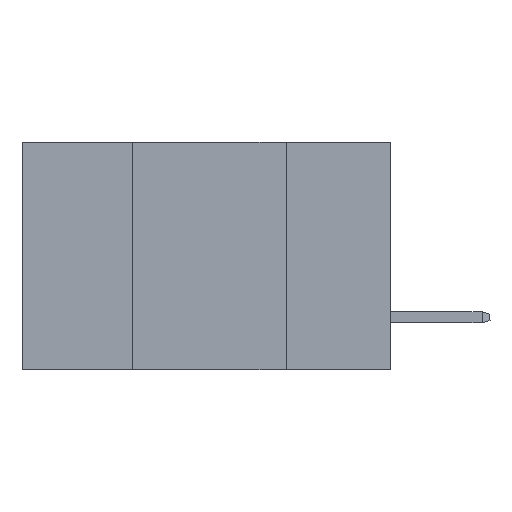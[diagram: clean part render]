
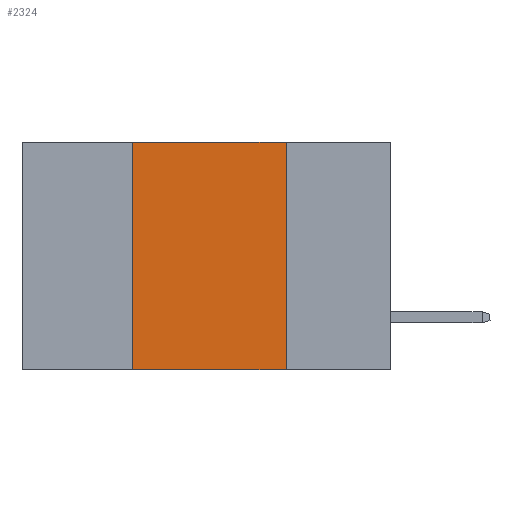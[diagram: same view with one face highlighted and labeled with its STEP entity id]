
A CAD part, left-side view. The second image highlights one B-rep face of the part: STEP entity #2324.
In plain terms, the highlighted planar face has unit normal (-1, 0, 0).
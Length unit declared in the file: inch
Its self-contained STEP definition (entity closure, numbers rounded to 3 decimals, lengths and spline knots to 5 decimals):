
#345 = VERTEX_POINT ( 'NONE', #1541 ) ;
#495 = VECTOR ( 'NONE', #648, 39.37008 ) ;
#512 = EDGE_LOOP ( 'NONE', ( #8416, #5565, #4851, #6882 ) ) ;
#648 = DIRECTION ( 'NONE',  ( 0., -1., 0. ) ) ;
#925 = CARTESIAN_POINT ( 'NONE',  ( 0., 0.17, 0. ) ) ;
#994 = CARTESIAN_POINT ( 'NONE',  ( 0., 0.42, 0. ) ) ;
#1031 = VECTOR ( 'NONE', #8140, 39.37008 ) ;
#1502 = LINE ( 'NONE', #4062, #2975 ) ;
#1541 = CARTESIAN_POINT ( 'NONE',  ( 0., 0.17, 0. ) ) ;
#1684 = VECTOR ( 'NONE', #4405, 39.37008 ) ;
#2297 = VERTEX_POINT ( 'NONE', #6514 ) ;
#2324 = ADVANCED_FACE ( 'NONE', ( #8362 ), #5560, .F. ) ;
#2580 = EDGE_CURVE ( 'NONE', #8582, #345, #1502, .T. ) ;
#2642 = CARTESIAN_POINT ( 'NONE',  ( 0., 0.6, -0.37 ) ) ;
#2975 = VECTOR ( 'NONE', #6668, 39.37008 ) ;
#3455 = EDGE_CURVE ( 'NONE', #345, #2297, #6512, .T. ) ;
#3498 = CARTESIAN_POINT ( 'NONE',  ( 0., 0.42, 0. ) ) ;
#4062 = CARTESIAN_POINT ( 'NONE',  ( 0., 0.6, 0. ) ) ;
#4255 = EDGE_CURVE ( 'NONE', #4478, #8582, #8702, .T. ) ;
#4405 = DIRECTION ( 'NONE',  ( 0., 0., 1. ) ) ;
#4478 = VERTEX_POINT ( 'NONE', #7391 ) ;
#4806 = AXIS2_PLACEMENT_3D ( 'NONE', #6916, #5547, #7185 ) ;
#4851 = ORIENTED_EDGE ( 'NONE', *, *, #4255, .F. ) ;
#5547 = DIRECTION ( 'NONE',  ( 1., 0., 0. ) ) ;
#5560 = PLANE ( 'NONE',  #4806 ) ;
#5565 = ORIENTED_EDGE ( 'NONE', *, *, #2580, .F. ) ;
#5833 = LINE ( 'NONE', #2642, #495 ) ;
#6512 = LINE ( 'NONE', #925, #1031 ) ;
#6514 = CARTESIAN_POINT ( 'NONE',  ( 0., 0.17, -0.37 ) ) ;
#6633 = EDGE_CURVE ( 'NONE', #4478, #2297, #5833, .T. ) ;
#6668 = DIRECTION ( 'NONE',  ( 0., -1., 0. ) ) ;
#6882 = ORIENTED_EDGE ( 'NONE', *, *, #6633, .T. ) ;
#6916 = CARTESIAN_POINT ( 'NONE',  ( 0., 0.6, 0. ) ) ;
#7185 = DIRECTION ( 'NONE',  ( 0., 0., -1. ) ) ;
#7391 = CARTESIAN_POINT ( 'NONE',  ( 0., 0.42, -0.37 ) ) ;
#8140 = DIRECTION ( 'NONE',  ( 0., 0., -1. ) ) ;
#8362 = FACE_OUTER_BOUND ( 'NONE', #512, .T. ) ;
#8416 = ORIENTED_EDGE ( 'NONE', *, *, #3455, .F. ) ;
#8582 = VERTEX_POINT ( 'NONE', #3498 ) ;
#8702 = LINE ( 'NONE', #994, #1684 ) ;
